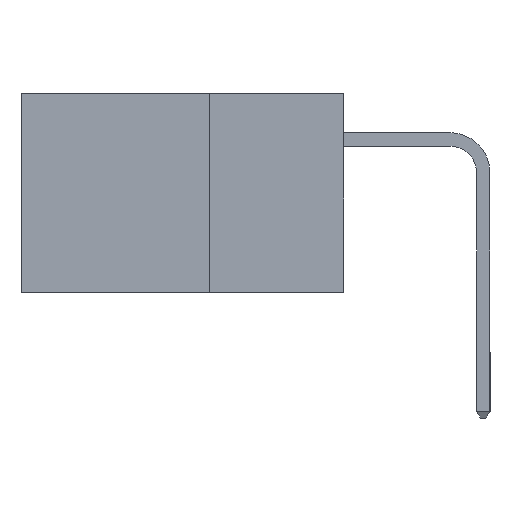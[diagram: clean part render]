
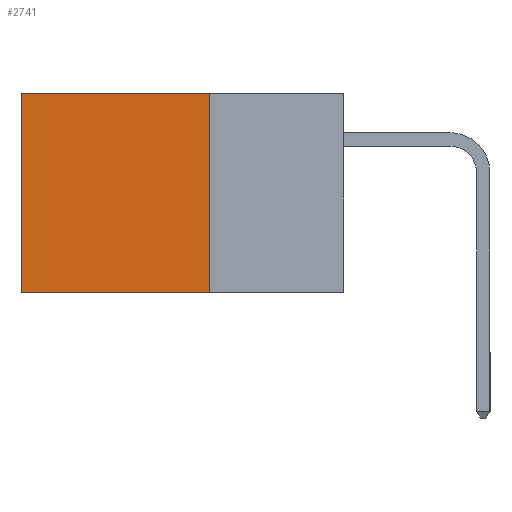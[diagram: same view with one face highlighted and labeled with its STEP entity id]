
A CAD part, left-side view. The second image highlights one B-rep face of the part: STEP entity #2741.
In plain terms, the highlighted planar face has unit normal (-1, 0, 0).
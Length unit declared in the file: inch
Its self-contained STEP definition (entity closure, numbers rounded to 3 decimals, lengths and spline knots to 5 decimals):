
#261 = EDGE_CURVE ( 'NONE', #3721, #7446, #11583, .T. ) ;
#266 = AXIS2_PLACEMENT_3D ( 'NONE', #2096, #11574, #7923 ) ;
#470 = CARTESIAN_POINT ( 'NONE',  ( 0.298, 0.6, 0. ) ) ;
#538 = DIRECTION ( 'NONE',  ( 0., 0., -1. ) ) ;
#1637 = CARTESIAN_POINT ( 'NONE',  ( 0.298, 0.25, -0.37 ) ) ;
#1643 = EDGE_LOOP ( 'NONE', ( #7161, #15175, #6643, #5664 ) ) ;
#1937 = EDGE_CURVE ( 'NONE', #13724, #2424, #13580, .T. ) ;
#2096 = CARTESIAN_POINT ( 'NONE',  ( 0.298, 0.25, 0. ) ) ;
#2424 = VERTEX_POINT ( 'NONE', #470 ) ;
#2741 = ADVANCED_FACE ( 'NONE', ( #13186 ), #7675, .F. ) ;
#3186 = CARTESIAN_POINT ( 'NONE',  ( 0.298, 0.6, -0.37 ) ) ;
#3721 = VERTEX_POINT ( 'NONE', #9721 ) ;
#4495 = VECTOR ( 'NONE', #538, 39.37008 ) ;
#4672 = DIRECTION ( 'NONE',  ( 0., 1., 0. ) ) ;
#5664 = ORIENTED_EDGE ( 'NONE', *, *, #1937, .T. ) ;
#6543 = EDGE_CURVE ( 'NONE', #13724, #3721, #12275, .T. ) ;
#6643 = ORIENTED_EDGE ( 'NONE', *, *, #6543, .F. ) ;
#7161 = ORIENTED_EDGE ( 'NONE', *, *, #11285, .T. ) ;
#7357 = DIRECTION ( 'NONE',  ( 0., 0., -1. ) ) ;
#7446 = VERTEX_POINT ( 'NONE', #3186 ) ;
#7675 = PLANE ( 'NONE',  #266 ) ;
#7923 = DIRECTION ( 'NONE',  ( 0., 0., -1. ) ) ;
#8291 = CARTESIAN_POINT ( 'NONE',  ( 0.298, 0.25, 0. ) ) ;
#8352 = VECTOR ( 'NONE', #4672, 39.37008 ) ;
#8531 = VECTOR ( 'NONE', #7357, 39.37008 ) ;
#9721 = CARTESIAN_POINT ( 'NONE',  ( 0.298, 0.25, -0.37 ) ) ;
#10327 = DIRECTION ( 'NONE',  ( 0., 1., 0. ) ) ;
#10886 = CARTESIAN_POINT ( 'NONE',  ( 0.298, 0.6, 0. ) ) ;
#11285 = EDGE_CURVE ( 'NONE', #2424, #7446, #12637, .T. ) ;
#11574 = DIRECTION ( 'NONE',  ( 1., 0., 0. ) ) ;
#11583 = LINE ( 'NONE', #1637, #11750 ) ;
#11750 = VECTOR ( 'NONE', #10327, 39.37008 ) ;
#12275 = LINE ( 'NONE', #13526, #4495 ) ;
#12637 = LINE ( 'NONE', #10886, #8531 ) ;
#13186 = FACE_OUTER_BOUND ( 'NONE', #1643, .T. ) ;
#13526 = CARTESIAN_POINT ( 'NONE',  ( 0.298, 0.25, 0. ) ) ;
#13580 = LINE ( 'NONE', #8291, #8352 ) ;
#13724 = VERTEX_POINT ( 'NONE', #15230 ) ;
#15175 = ORIENTED_EDGE ( 'NONE', *, *, #261, .F. ) ;
#15230 = CARTESIAN_POINT ( 'NONE',  ( 0.298, 0.25, 0. ) ) ;
